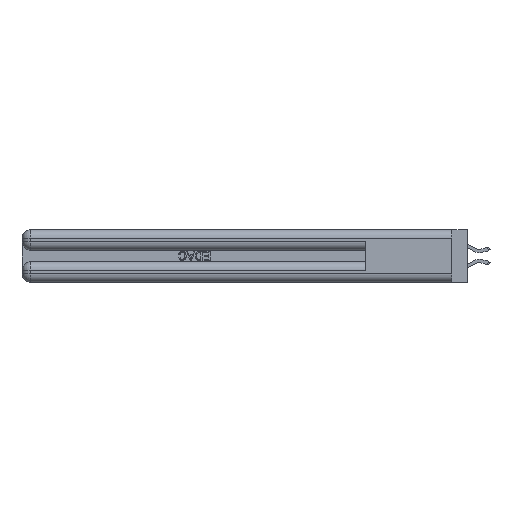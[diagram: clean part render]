
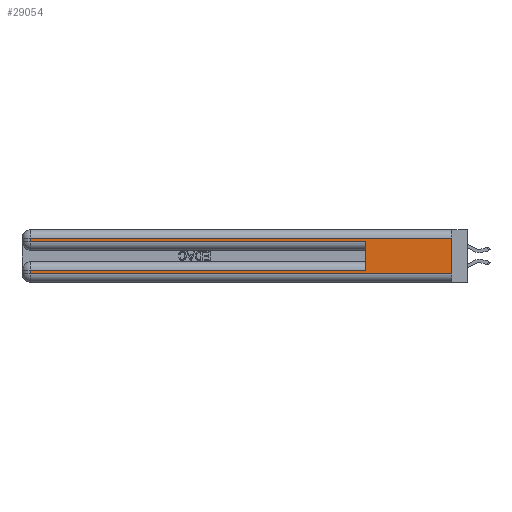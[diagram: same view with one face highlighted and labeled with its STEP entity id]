
A CAD part, left-side view. The second image highlights one B-rep face of the part: STEP entity #29054.
In plain terms, the highlighted planar face has unit normal (-1, 0, 0).
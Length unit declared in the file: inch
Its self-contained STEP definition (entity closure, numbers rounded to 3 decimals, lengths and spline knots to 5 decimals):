
#679 = CARTESIAN_POINT ( 'NONE',  ( 0., 0., 0.06 ) ) ;
#899 = ORIENTED_EDGE ( 'NONE', *, *, #9847, .T. ) ;
#1447 = DIRECTION ( 'NONE',  ( 1., 0., 0. ) ) ;
#1668 = LINE ( 'NONE', #5685, #15459 ) ;
#2920 = VECTOR ( 'NONE', #6569, 39.37008 ) ;
#3069 = CARTESIAN_POINT ( 'NONE',  ( 0., 0., 0.31 ) ) ;
#3658 = VECTOR ( 'NONE', #6449, 39.37008 ) ;
#4258 = PLANE ( 'NONE',  #35206 ) ;
#4464 = EDGE_CURVE ( 'NONE', #11903, #27737, #1668, .T. ) ;
#4592 = EDGE_CURVE ( 'NONE', #27562, #20863, #25533, .T. ) ;
#5145 = FACE_OUTER_BOUND ( 'NONE', #32498, .T. ) ;
#5158 = LINE ( 'NONE', #13363, #25370 ) ;
#5448 = EDGE_CURVE ( 'NONE', #20863, #23402, #37719, .T. ) ;
#5592 = ORIENTED_EDGE ( 'NONE', *, *, #4464, .T. ) ;
#5685 = CARTESIAN_POINT ( 'NONE',  ( 0., 0., 0.085 ) ) ;
#6012 = CARTESIAN_POINT ( 'NONE',  ( 0., 2.94, 0.37 ) ) ;
#6383 = ORIENTED_EDGE ( 'NONE', *, *, #5448, .T. ) ;
#6449 = DIRECTION ( 'NONE',  ( 0., -1., 0. ) ) ;
#6569 = DIRECTION ( 'NONE',  ( 0., -1., 0. ) ) ;
#6583 = LINE ( 'NONE', #679, #2920 ) ;
#6626 = VECTOR ( 'NONE', #15119, 39.37008 ) ;
#6812 = ORIENTED_EDGE ( 'NONE', *, *, #4592, .T. ) ;
#7520 = DIRECTION ( 'NONE',  ( 0., 0., -1. ) ) ;
#8171 = ORIENTED_EDGE ( 'NONE', *, *, #21227, .T. ) ;
#9421 = ORIENTED_EDGE ( 'NONE', *, *, #16698, .F. ) ;
#9847 = EDGE_CURVE ( 'NONE', #36444, #31364, #6583, .T. ) ;
#10370 = CARTESIAN_POINT ( 'NONE',  ( 0., 0., 0.37 ) ) ;
#11539 = CARTESIAN_POINT ( 'NONE',  ( 0., 2.94, 0.06 ) ) ;
#11704 = EDGE_CURVE ( 'NONE', #27562, #31364, #28886, .T. ) ;
#11903 = VERTEX_POINT ( 'NONE', #20253 ) ;
#12069 = DIRECTION ( 'NONE',  ( 0., 1., 0. ) ) ;
#12638 = CARTESIAN_POINT ( 'NONE',  ( 0., 2.94, 0.085 ) ) ;
#13363 = CARTESIAN_POINT ( 'NONE',  ( 0., 0.6, 0.145 ) ) ;
#13677 = CARTESIAN_POINT ( 'NONE',  ( 0., 2.94, 0.31 ) ) ;
#14384 = CARTESIAN_POINT ( 'NONE',  ( 0., 2.94, 0.285 ) ) ;
#15119 = DIRECTION ( 'NONE',  ( 0., 0., -1. ) ) ;
#15459 = VECTOR ( 'NONE', #12069, 39.37008 ) ;
#16698 = EDGE_CURVE ( 'NONE', #11903, #19210, #5158, .T. ) ;
#17468 = CARTESIAN_POINT ( 'NONE',  ( 0., 0., 0.06 ) ) ;
#17502 = CARTESIAN_POINT ( 'NONE',  ( 0., 0., 0.285 ) ) ;
#18008 = ORIENTED_EDGE ( 'NONE', *, *, #30371, .T. ) ;
#19210 = VERTEX_POINT ( 'NONE', #35925 ) ;
#20253 = CARTESIAN_POINT ( 'NONE',  ( 0., 0.6, 0.085 ) ) ;
#20374 = ORIENTED_EDGE ( 'NONE', *, *, #11704, .F. ) ;
#20462 = VECTOR ( 'NONE', #27312, 39.37008 ) ;
#20863 = VERTEX_POINT ( 'NONE', #13677 ) ;
#21227 = EDGE_CURVE ( 'NONE', #23402, #19210, #32508, .T. ) ;
#22111 = CARTESIAN_POINT ( 'NONE',  ( 0., 0., 0.37 ) ) ;
#22497 = LINE ( 'NONE', #27726, #25708 ) ;
#23402 = VERTEX_POINT ( 'NONE', #14384 ) ;
#24572 = DIRECTION ( 'NONE',  ( 0., 0., -1. ) ) ;
#24849 = DIRECTION ( 'NONE',  ( 0., 0., -1. ) ) ;
#25370 = VECTOR ( 'NONE', #33509, 39.37008 ) ;
#25533 = LINE ( 'NONE', #3069, #20462 ) ;
#25708 = VECTOR ( 'NONE', #24849, 39.37008 ) ;
#26979 = CARTESIAN_POINT ( 'NONE',  ( 0., 0., 0.31 ) ) ;
#27060 = VECTOR ( 'NONE', #7520, 39.37008 ) ;
#27312 = DIRECTION ( 'NONE',  ( 0., 1., 0. ) ) ;
#27562 = VERTEX_POINT ( 'NONE', #26979 ) ;
#27726 = CARTESIAN_POINT ( 'NONE',  ( 0., 2.94, 0.37 ) ) ;
#27737 = VERTEX_POINT ( 'NONE', #12638 ) ;
#28886 = LINE ( 'NONE', #10370, #27060 ) ;
#29054 = ADVANCED_FACE ( 'NONE', ( #5145 ), #4258, .F. ) ;
#30371 = EDGE_CURVE ( 'NONE', #27737, #36444, #22497, .T. ) ;
#31364 = VERTEX_POINT ( 'NONE', #17468 ) ;
#32498 = EDGE_LOOP ( 'NONE', ( #20374, #6812, #6383, #8171, #9421, #5592, #18008, #899 ) ) ;
#32508 = LINE ( 'NONE', #17502, #3658 ) ;
#33509 = DIRECTION ( 'NONE',  ( 0., 0., 1. ) ) ;
#35206 = AXIS2_PLACEMENT_3D ( 'NONE', #22111, #1447, #24572 ) ;
#35925 = CARTESIAN_POINT ( 'NONE',  ( 0., 0.6, 0.285 ) ) ;
#36444 = VERTEX_POINT ( 'NONE', #11539 ) ;
#37719 = LINE ( 'NONE', #6012, #6626 ) ;
